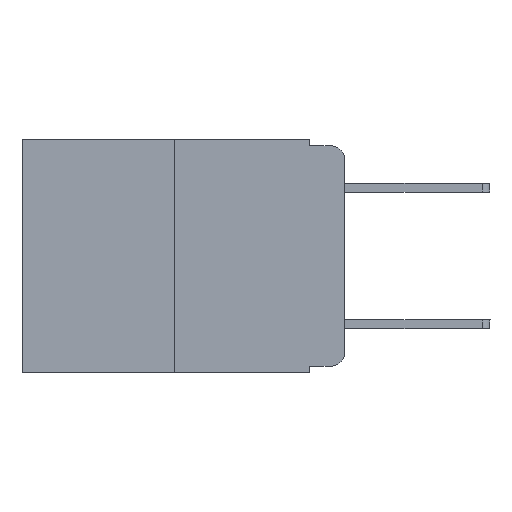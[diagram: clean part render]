
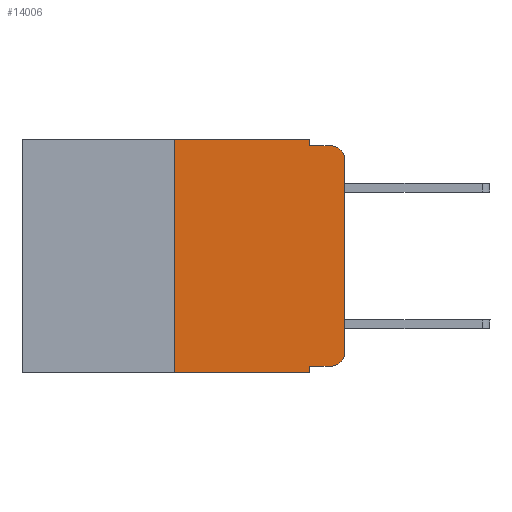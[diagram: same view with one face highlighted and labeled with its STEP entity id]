
A CAD part, left-side view. The second image highlights one B-rep face of the part: STEP entity #14006.
In plain terms, the highlighted planar face has unit normal (-1, 0, 0).
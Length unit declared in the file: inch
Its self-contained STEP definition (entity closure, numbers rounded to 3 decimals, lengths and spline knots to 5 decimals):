
#135 = VECTOR ( 'NONE', #17181, 39.37008 ) ;
#533 = EDGE_CURVE ( 'NONE', #15829, #15751, #16374, .T. ) ;
#883 = VECTOR ( 'NONE', #8847, 39.37008 ) ;
#1094 = CIRCLE ( 'NONE', #10523, 0.02 ) ;
#1347 = CARTESIAN_POINT ( 'NONE',  ( 0., 0.473, 0. ) ) ;
#1501 = ORIENTED_EDGE ( 'NONE', *, *, #4089, .T. ) ;
#1947 = DIRECTION ( 'NONE',  ( 0., 0., -1. ) ) ;
#2032 = DIRECTION ( 'NONE',  ( 0., -1., 0. ) ) ;
#2115 = CARTESIAN_POINT ( 'NONE',  ( 0., 0.051, 0. ) ) ;
#2161 = DIRECTION ( 'NONE',  ( 0., 0., -1. ) ) ;
#2741 = EDGE_CURVE ( 'NONE', #9983, #18219, #14846, .T. ) ;
#2802 = VECTOR ( 'NONE', #1947, 39.37008 ) ;
#3139 = EDGE_CURVE ( 'NONE', #7089, #15829, #8790, .T. ) ;
#3509 = CARTESIAN_POINT ( 'NONE',  ( 0., 0., -0.03 ) ) ;
#4089 = EDGE_CURVE ( 'NONE', #12603, #18219, #1094, .T. ) ;
#4371 = LINE ( 'NONE', #13531, #883 ) ;
#4892 = LINE ( 'NONE', #7850, #2802 ) ;
#5546 = DIRECTION ( 'NONE',  ( 0., -1., 0. ) ) ;
#5961 = LINE ( 'NONE', #14076, #14359 ) ;
#6089 = ORIENTED_EDGE ( 'NONE', *, *, #15405, .F. ) ;
#6113 = EDGE_CURVE ( 'NONE', #6795, #11757, #15998, .T. ) ;
#6305 = CARTESIAN_POINT ( 'NONE',  ( 0., 0.051, -0.01 ) ) ;
#6336 = ORIENTED_EDGE ( 'NONE', *, *, #2741, .F. ) ;
#6435 = CARTESIAN_POINT ( 'NONE',  ( 0., 0.25, 0. ) ) ;
#6547 = EDGE_CURVE ( 'NONE', #11262, #6795, #11367, .T. ) ;
#6670 = CARTESIAN_POINT ( 'NONE',  ( 0., 0.473, -0.343 ) ) ;
#6795 = VERTEX_POINT ( 'NONE', #6435 ) ;
#7089 = VERTEX_POINT ( 'NONE', #8959 ) ;
#7850 = CARTESIAN_POINT ( 'NONE',  ( 0., 0.051, 0. ) ) ;
#8364 = VERTEX_POINT ( 'NONE', #13747 ) ;
#8513 = EDGE_CURVE ( 'NONE', #15751, #12603, #4371, .T. ) ;
#8790 = LINE ( 'NONE', #15014, #135 ) ;
#8847 = DIRECTION ( 'NONE',  ( 0., 0., 1. ) ) ;
#8959 = CARTESIAN_POINT ( 'NONE',  ( 0., 0.051, -0.333 ) ) ;
#8980 = PLANE ( 'NONE',  #16986 ) ;
#9169 = EDGE_CURVE ( 'NONE', #11262, #8364, #19507, .T. ) ;
#9181 = DIRECTION ( 'NONE',  ( 0., 0., -1. ) ) ;
#9983 = VERTEX_POINT ( 'NONE', #6305 ) ;
#10523 = AXIS2_PLACEMENT_3D ( 'NONE', #16944, #15719, #9181 ) ;
#10978 = ORIENTED_EDGE ( 'NONE', *, *, #16764, .F. ) ;
#11262 = VERTEX_POINT ( 'NONE', #15060 ) ;
#11367 = LINE ( 'NONE', #12886, #13181 ) ;
#11757 = VERTEX_POINT ( 'NONE', #2115 ) ;
#11786 = EDGE_LOOP ( 'NONE', ( #13784, #1501, #6336, #10978, #19097, #15756, #18552, #6089, #13921, #17429 ) ) ;
#12603 = VERTEX_POINT ( 'NONE', #3509 ) ;
#12886 = CARTESIAN_POINT ( 'NONE',  ( 0., 0.25, 0. ) ) ;
#12947 = CARTESIAN_POINT ( 'NONE',  ( 0., 0.02, -0.313 ) ) ;
#13122 = CARTESIAN_POINT ( 'NONE',  ( 0., 0.02, -0.01 ) ) ;
#13181 = VECTOR ( 'NONE', #16165, 39.37008 ) ;
#13310 = DIRECTION ( 'NONE',  ( 0., -1., 0. ) ) ;
#13531 = CARTESIAN_POINT ( 'NONE',  ( 0., 0., 0. ) ) ;
#13747 = CARTESIAN_POINT ( 'NONE',  ( 0., 0.051, -0.343 ) ) ;
#13784 = ORIENTED_EDGE ( 'NONE', *, *, #8513, .T. ) ;
#13921 = ORIENTED_EDGE ( 'NONE', *, *, #3139, .T. ) ;
#14006 = ADVANCED_FACE ( 'NONE', ( #16841 ), #8980, .F. ) ;
#14076 = CARTESIAN_POINT ( 'NONE',  ( 0., 0.051, 0. ) ) ;
#14359 = VECTOR ( 'NONE', #17348, 39.37008 ) ;
#14846 = LINE ( 'NONE', #19716, #16828 ) ;
#14987 = CARTESIAN_POINT ( 'NONE',  ( 0., 0., -0.313 ) ) ;
#15014 = CARTESIAN_POINT ( 'NONE',  ( 0., 0.051, -0.333 ) ) ;
#15060 = CARTESIAN_POINT ( 'NONE',  ( 0., 0.25, -0.343 ) ) ;
#15200 = DIRECTION ( 'NONE',  ( 1., 0., 0. ) ) ;
#15405 = EDGE_CURVE ( 'NONE', #7089, #8364, #5961, .T. ) ;
#15719 = DIRECTION ( 'NONE',  ( -1., 0., 0. ) ) ;
#15751 = VERTEX_POINT ( 'NONE', #14987 ) ;
#15756 = ORIENTED_EDGE ( 'NONE', *, *, #6547, .F. ) ;
#15829 = VERTEX_POINT ( 'NONE', #19011 ) ;
#15998 = LINE ( 'NONE', #17715, #18055 ) ;
#16122 = DIRECTION ( 'NONE',  ( -1., 0., 0. ) ) ;
#16165 = DIRECTION ( 'NONE',  ( 0., 0., 1. ) ) ;
#16230 = VECTOR ( 'NONE', #5546, 39.37008 ) ;
#16374 = CIRCLE ( 'NONE', #18336, 0.02 ) ;
#16764 = EDGE_CURVE ( 'NONE', #11757, #9983, #4892, .T. ) ;
#16828 = VECTOR ( 'NONE', #13310, 39.37008 ) ;
#16841 = FACE_OUTER_BOUND ( 'NONE', #11786, .T. ) ;
#16944 = CARTESIAN_POINT ( 'NONE',  ( 0., 0.02, -0.03 ) ) ;
#16986 = AXIS2_PLACEMENT_3D ( 'NONE', #1347, #15200, #19884 ) ;
#17181 = DIRECTION ( 'NONE',  ( 0., -1., 0. ) ) ;
#17348 = DIRECTION ( 'NONE',  ( 0., 0., -1. ) ) ;
#17429 = ORIENTED_EDGE ( 'NONE', *, *, #533, .T. ) ;
#17715 = CARTESIAN_POINT ( 'NONE',  ( 0., 0.473, 0. ) ) ;
#18055 = VECTOR ( 'NONE', #2032, 39.37008 ) ;
#18219 = VERTEX_POINT ( 'NONE', #13122 ) ;
#18336 = AXIS2_PLACEMENT_3D ( 'NONE', #12947, #16122, #2161 ) ;
#18552 = ORIENTED_EDGE ( 'NONE', *, *, #9169, .T. ) ;
#19011 = CARTESIAN_POINT ( 'NONE',  ( 0., 0.02, -0.333 ) ) ;
#19097 = ORIENTED_EDGE ( 'NONE', *, *, #6113, .F. ) ;
#19507 = LINE ( 'NONE', #6670, #16230 ) ;
#19716 = CARTESIAN_POINT ( 'NONE',  ( 0., 0.051, -0.01 ) ) ;
#19884 = DIRECTION ( 'NONE',  ( 0., 0., -1. ) ) ;
